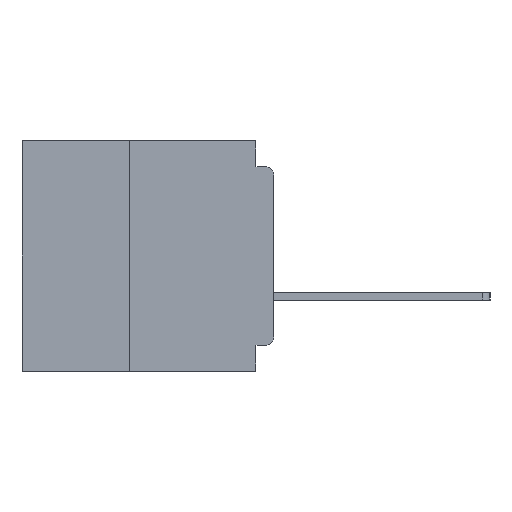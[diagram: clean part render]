
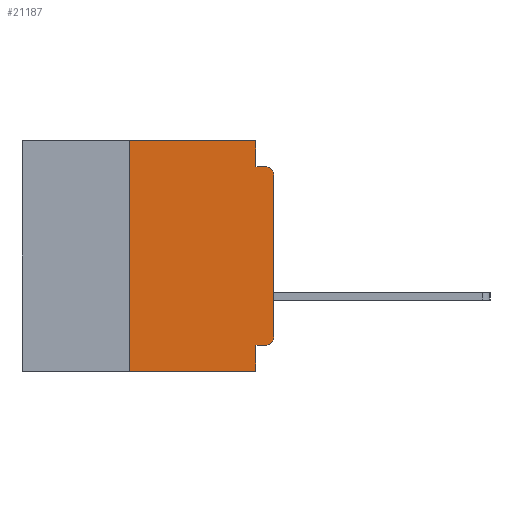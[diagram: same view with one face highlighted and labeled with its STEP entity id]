
A CAD part, left-side view. The second image highlights one B-rep face of the part: STEP entity #21187.
In plain terms, the highlighted planar face has unit normal (-1, 0, 0).
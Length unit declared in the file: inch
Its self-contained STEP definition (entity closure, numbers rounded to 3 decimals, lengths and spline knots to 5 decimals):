
#689 = EDGE_CURVE ( 'NONE', #43089, #42025, #17841, .T. ) ;
#1295 = VECTOR ( 'NONE', #19176, 39.37008 ) ;
#2095 = CARTESIAN_POINT ( 'NONE',  ( 0., 0., -0.355 ) ) ;
#2417 = VERTEX_POINT ( 'NONE', #8488 ) ;
#2422 = DIRECTION ( 'NONE',  ( 0., 0., -1. ) ) ;
#4104 = CARTESIAN_POINT ( 'NONE',  ( 0., 0.25, -0.4 ) ) ;
#4369 = ORIENTED_EDGE ( 'NONE', *, *, #16451, .T. ) ;
#4376 = CARTESIAN_POINT ( 'NONE',  ( 0., 0.25, -0.4 ) ) ;
#4917 = CARTESIAN_POINT ( 'NONE',  ( 0., 0.031, 0. ) ) ;
#5414 = DIRECTION ( 'NONE',  ( 1., 0., 0. ) ) ;
#7057 = CIRCLE ( 'NONE', #36101, 0.015 ) ;
#8488 = CARTESIAN_POINT ( 'NONE',  ( 0., 0.015, -0.355 ) ) ;
#8713 = CARTESIAN_POINT ( 'NONE',  ( 0., 0., -0.34 ) ) ;
#9172 = ORIENTED_EDGE ( 'NONE', *, *, #29106, .F. ) ;
#10351 = ORIENTED_EDGE ( 'NONE', *, *, #32360, .F. ) ;
#10942 = CARTESIAN_POINT ( 'NONE',  ( 0., 0.437, -0.4 ) ) ;
#10982 = EDGE_CURVE ( 'NONE', #21739, #44311, #33059, .T. ) ;
#11503 = CARTESIAN_POINT ( 'NONE',  ( 0., 0., 0. ) ) ;
#11993 = DIRECTION ( 'NONE',  ( 0., -1., 0. ) ) ;
#12809 = DIRECTION ( 'NONE',  ( 0., 0., -1. ) ) ;
#12971 = CIRCLE ( 'NONE', #25539, 0.015 ) ;
#14590 = DIRECTION ( 'NONE',  ( -1., 0., 0. ) ) ;
#16451 = EDGE_CURVE ( 'NONE', #38921, #19653, #26035, .T. ) ;
#17013 = LINE ( 'NONE', #34888, #25991 ) ;
#17841 = LINE ( 'NONE', #43481, #29220 ) ;
#18456 = VECTOR ( 'NONE', #44132, 39.37008 ) ;
#18907 = CARTESIAN_POINT ( 'NONE',  ( 0., 0.015, -0.045 ) ) ;
#19176 = DIRECTION ( 'NONE',  ( 0., 0., 1. ) ) ;
#19297 = ORIENTED_EDGE ( 'NONE', *, *, #29907, .T. ) ;
#19653 = VERTEX_POINT ( 'NONE', #19849 ) ;
#19744 = EDGE_CURVE ( 'NONE', #42025, #40913, #38903, .T. ) ;
#19849 = CARTESIAN_POINT ( 'NONE',  ( 0., 0.031, -0.4 ) ) ;
#19926 = ORIENTED_EDGE ( 'NONE', *, *, #689, .F. ) ;
#20517 = DIRECTION ( 'NONE',  ( 0., -1., 0. ) ) ;
#20547 = ORIENTED_EDGE ( 'NONE', *, *, #29159, .T. ) ;
#21187 = ADVANCED_FACE ( 'NONE', ( #31299 ), #28360, .F. ) ;
#21739 = VERTEX_POINT ( 'NONE', #8713 ) ;
#22302 = CARTESIAN_POINT ( 'NONE',  ( 0., 0.031, 0. ) ) ;
#23597 = VECTOR ( 'NONE', #45421, 39.37008 ) ;
#23885 = VERTEX_POINT ( 'NONE', #18907 ) ;
#24600 = EDGE_LOOP ( 'NONE', ( #36082, #19297, #10351, #35481, #19926, #43926, #4369, #34893, #9172, #20547 ) ) ;
#25350 = DIRECTION ( 'NONE',  ( -1., 0., 0. ) ) ;
#25539 = AXIS2_PLACEMENT_3D ( 'NONE', #37533, #14590, #41395 ) ;
#25932 = AXIS2_PLACEMENT_3D ( 'NONE', #47433, #5414, #32215 ) ;
#25991 = VECTOR ( 'NONE', #11993, 39.37008 ) ;
#26035 = LINE ( 'NONE', #10942, #23597 ) ;
#27489 = VECTOR ( 'NONE', #12809, 39.37008 ) ;
#28360 = PLANE ( 'NONE',  #25932 ) ;
#29106 = EDGE_CURVE ( 'NONE', #2417, #29693, #40029, .T. ) ;
#29159 = EDGE_CURVE ( 'NONE', #2417, #21739, #7057, .T. ) ;
#29220 = VECTOR ( 'NONE', #20517, 39.37008 ) ;
#29693 = VERTEX_POINT ( 'NONE', #43909 ) ;
#29907 = EDGE_CURVE ( 'NONE', #44311, #23885, #12971, .T. ) ;
#31299 = FACE_OUTER_BOUND ( 'NONE', #24600, .T. ) ;
#31481 = CARTESIAN_POINT ( 'NONE',  ( 0., 0., -0.06 ) ) ;
#31678 = CARTESIAN_POINT ( 'NONE',  ( 0., 0.031, -0.4 ) ) ;
#32215 = DIRECTION ( 'NONE',  ( 0., 0., -1. ) ) ;
#32360 = EDGE_CURVE ( 'NONE', #40913, #23885, #17013, .T. ) ;
#33059 = LINE ( 'NONE', #11503, #1295 ) ;
#34572 = VECTOR ( 'NONE', #34987, 39.37008 ) ;
#34888 = CARTESIAN_POINT ( 'NONE',  ( 0., 0., -0.045 ) ) ;
#34893 = ORIENTED_EDGE ( 'NONE', *, *, #41649, .F. ) ;
#34987 = DIRECTION ( 'NONE',  ( 0., 0., 1. ) ) ;
#35443 = CARTESIAN_POINT ( 'NONE',  ( 0., 0.25, 0. ) ) ;
#35481 = ORIENTED_EDGE ( 'NONE', *, *, #19744, .F. ) ;
#35626 = VECTOR ( 'NONE', #47060, 39.37008 ) ;
#36082 = ORIENTED_EDGE ( 'NONE', *, *, #10982, .T. ) ;
#36101 = AXIS2_PLACEMENT_3D ( 'NONE', #48274, #25350, #2422 ) ;
#37533 = CARTESIAN_POINT ( 'NONE',  ( 0., 0.015, -0.06 ) ) ;
#38607 = CARTESIAN_POINT ( 'NONE',  ( 0., 0.031, -0.045 ) ) ;
#38903 = LINE ( 'NONE', #4917, #27489 ) ;
#38921 = VERTEX_POINT ( 'NONE', #4104 ) ;
#40029 = LINE ( 'NONE', #2095, #18456 ) ;
#40913 = VERTEX_POINT ( 'NONE', #38607 ) ;
#41395 = DIRECTION ( 'NONE',  ( 0., 0., -1. ) ) ;
#41649 = EDGE_CURVE ( 'NONE', #29693, #19653, #45840, .T. ) ;
#42025 = VERTEX_POINT ( 'NONE', #22302 ) ;
#43089 = VERTEX_POINT ( 'NONE', #35443 ) ;
#43481 = CARTESIAN_POINT ( 'NONE',  ( 0., 0.437, 0. ) ) ;
#43909 = CARTESIAN_POINT ( 'NONE',  ( 0., 0.031, -0.355 ) ) ;
#43926 = ORIENTED_EDGE ( 'NONE', *, *, #44267, .F. ) ;
#44132 = DIRECTION ( 'NONE',  ( 0., 1., 0. ) ) ;
#44267 = EDGE_CURVE ( 'NONE', #38921, #43089, #44813, .T. ) ;
#44311 = VERTEX_POINT ( 'NONE', #31481 ) ;
#44813 = LINE ( 'NONE', #4376, #34572 ) ;
#45421 = DIRECTION ( 'NONE',  ( 0., -1., 0. ) ) ;
#45840 = LINE ( 'NONE', #31678, #35626 ) ;
#47060 = DIRECTION ( 'NONE',  ( 0., 0., -1. ) ) ;
#47433 = CARTESIAN_POINT ( 'NONE',  ( 0., 0.437, 0. ) ) ;
#48274 = CARTESIAN_POINT ( 'NONE',  ( 0., 0.015, -0.34 ) ) ;
